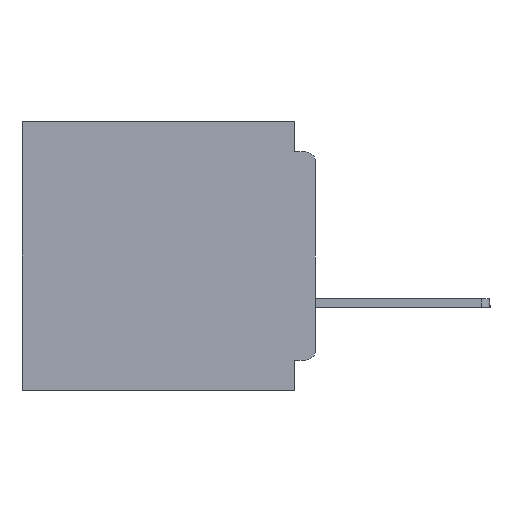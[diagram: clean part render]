
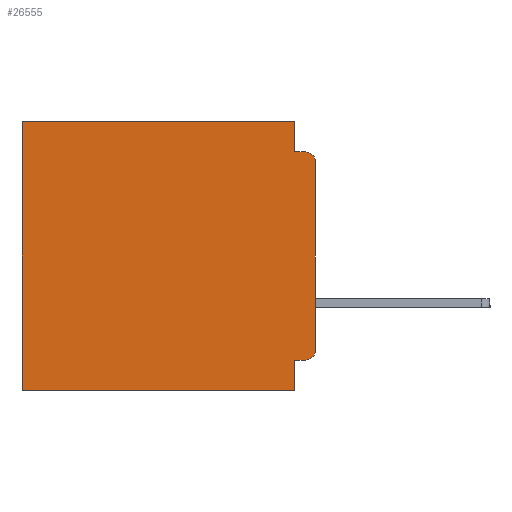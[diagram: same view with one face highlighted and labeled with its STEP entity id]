
A CAD part, left-side view. The second image highlights one B-rep face of the part: STEP entity #26555.
In plain terms, the highlighted planar face has unit normal (-1, 0, 0).
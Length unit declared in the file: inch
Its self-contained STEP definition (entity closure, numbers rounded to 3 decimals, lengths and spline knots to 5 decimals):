
#454 = CARTESIAN_POINT ( 'NONE',  ( 0.3, 0.015, -0.355 ) ) ;
#2407 = ORIENTED_EDGE ( 'NONE', *, *, #19476, .T. ) ;
#2650 = ORIENTED_EDGE ( 'NONE', *, *, #13408, .F. ) ;
#4534 = VECTOR ( 'NONE', #26226, 39.37008 ) ;
#4838 = ORIENTED_EDGE ( 'NONE', *, *, #21185, .T. ) ;
#4865 = VECTOR ( 'NONE', #31657, 39.37008 ) ;
#5301 = EDGE_LOOP ( 'NONE', ( #19419, #4838, #31315, #20966, #7422, #2407, #13477, #11818, #2650, #13776 ) ) ;
#5565 = CARTESIAN_POINT ( 'NONE',  ( 0.3, 0.031, -0.4 ) ) ;
#6075 = EDGE_CURVE ( 'NONE', #13220, #10098, #6987, .T. ) ;
#6446 = AXIS2_PLACEMENT_3D ( 'NONE', #13813, #32935, #16598 ) ;
#6987 = LINE ( 'NONE', #28597, #33619 ) ;
#7422 = ORIENTED_EDGE ( 'NONE', *, *, #6075, .T. ) ;
#8342 = DIRECTION ( 'NONE',  ( 0., 0., -1. ) ) ;
#8594 = VECTOR ( 'NONE', #16568, 39.37008 ) ;
#8645 = CARTESIAN_POINT ( 'NONE',  ( 0.3, 0.437, 0. ) ) ;
#9035 = FACE_OUTER_BOUND ( 'NONE', #5301, .T. ) ;
#9149 = CARTESIAN_POINT ( 'NONE',  ( 0.3, 0., -0.34 ) ) ;
#9679 = EDGE_CURVE ( 'NONE', #10384, #25102, #25056, .T. ) ;
#9707 = CARTESIAN_POINT ( 'NONE',  ( 0.3, 0.031, 0. ) ) ;
#10018 = CARTESIAN_POINT ( 'NONE',  ( 0.3, 0.437, -0.4 ) ) ;
#10098 = VERTEX_POINT ( 'NONE', #8645 ) ;
#10384 = VERTEX_POINT ( 'NONE', #29131 ) ;
#10449 = VECTOR ( 'NONE', #8342, 39.37008 ) ;
#11198 = LINE ( 'NONE', #32913, #8594 ) ;
#11327 = VECTOR ( 'NONE', #35413, 39.37008 ) ;
#11402 = DIRECTION ( 'NONE',  ( -1., 0., 0. ) ) ;
#11818 = ORIENTED_EDGE ( 'NONE', *, *, #19840, .F. ) ;
#11869 = LINE ( 'NONE', #31693, #4534 ) ;
#12404 = CARTESIAN_POINT ( 'NONE',  ( 0.3, 0., -0.4 ) ) ;
#13014 = LINE ( 'NONE', #15460, #20321 ) ;
#13047 = CARTESIAN_POINT ( 'NONE',  ( 0.3, 0., -0.4 ) ) ;
#13220 = VERTEX_POINT ( 'NONE', #34909 ) ;
#13408 = EDGE_CURVE ( 'NONE', #24658, #20834, #11198, .T. ) ;
#13477 = ORIENTED_EDGE ( 'NONE', *, *, #19464, .F. ) ;
#13776 = ORIENTED_EDGE ( 'NONE', *, *, #18913, .T. ) ;
#13813 = CARTESIAN_POINT ( 'NONE',  ( 0.3, 0.015, -0.06 ) ) ;
#13959 = LINE ( 'NONE', #9707, #4865 ) ;
#15460 = CARTESIAN_POINT ( 'NONE',  ( 0.3, 0.031, -0.4 ) ) ;
#15834 = DIRECTION ( 'NONE',  ( 0., 0., -1. ) ) ;
#16134 = VERTEX_POINT ( 'NONE', #29648 ) ;
#16568 = DIRECTION ( 'NONE',  ( 0., 1., 0. ) ) ;
#16598 = DIRECTION ( 'NONE',  ( 0., 0., -1. ) ) ;
#17477 = VERTEX_POINT ( 'NONE', #10018 ) ;
#17479 = AXIS2_PLACEMENT_3D ( 'NONE', #27845, #11402, #30570 ) ;
#18207 = VERTEX_POINT ( 'NONE', #5565 ) ;
#18913 = EDGE_CURVE ( 'NONE', #24658, #25102, #24112, .T. ) ;
#19419 = ORIENTED_EDGE ( 'NONE', *, *, #9679, .F. ) ;
#19464 = EDGE_CURVE ( 'NONE', #18207, #17477, #34023, .T. ) ;
#19476 = EDGE_CURVE ( 'NONE', #10098, #17477, #25930, .T. ) ;
#19840 = EDGE_CURVE ( 'NONE', #20834, #18207, #13014, .T. ) ;
#20321 = VECTOR ( 'NONE', #23673, 39.37008 ) ;
#20834 = VERTEX_POINT ( 'NONE', #31271 ) ;
#20966 = ORIENTED_EDGE ( 'NONE', *, *, #32273, .F. ) ;
#21185 = EDGE_CURVE ( 'NONE', #10384, #26881, #31320, .T. ) ;
#22052 = CARTESIAN_POINT ( 'NONE',  ( 0.3, 0.437, -0.4 ) ) ;
#23673 = DIRECTION ( 'NONE',  ( 0., 0., -1. ) ) ;
#23947 = PLANE ( 'NONE',  #27771 ) ;
#24112 = CIRCLE ( 'NONE', #17479, 0.015 ) ;
#24658 = VERTEX_POINT ( 'NONE', #454 ) ;
#25056 = LINE ( 'NONE', #12404, #33185 ) ;
#25102 = VERTEX_POINT ( 'NONE', #9149 ) ;
#25930 = LINE ( 'NONE', #22052, #10449 ) ;
#26226 = DIRECTION ( 'NONE',  ( 0., -1., 0. ) ) ;
#26555 = ADVANCED_FACE ( 'NONE', ( #9035 ), #23947, .F. ) ;
#26881 = VERTEX_POINT ( 'NONE', #30743 ) ;
#27771 = AXIS2_PLACEMENT_3D ( 'NONE', #13047, #32179, #15834 ) ;
#27845 = CARTESIAN_POINT ( 'NONE',  ( 0.3, 0.015, -0.34 ) ) ;
#28597 = CARTESIAN_POINT ( 'NONE',  ( 0.3, 0., 0. ) ) ;
#29131 = CARTESIAN_POINT ( 'NONE',  ( 0.3, 0., -0.06 ) ) ;
#29648 = CARTESIAN_POINT ( 'NONE',  ( 0.3, 0.031, -0.045 ) ) ;
#29965 = EDGE_CURVE ( 'NONE', #16134, #26881, #11869, .T. ) ;
#30174 = CARTESIAN_POINT ( 'NONE',  ( 0.3, 0., -0.4 ) ) ;
#30570 = DIRECTION ( 'NONE',  ( 0., 0., -1. ) ) ;
#30743 = CARTESIAN_POINT ( 'NONE',  ( 0.3, 0.015, -0.045 ) ) ;
#31271 = CARTESIAN_POINT ( 'NONE',  ( 0.3, 0.031, -0.355 ) ) ;
#31315 = ORIENTED_EDGE ( 'NONE', *, *, #29965, .F. ) ;
#31320 = CIRCLE ( 'NONE', #6446, 0.015 ) ;
#31338 = DIRECTION ( 'NONE',  ( 0., 1., 0. ) ) ;
#31556 = DIRECTION ( 'NONE',  ( 0., 0., -1. ) ) ;
#31657 = DIRECTION ( 'NONE',  ( 0., 0., -1. ) ) ;
#31693 = CARTESIAN_POINT ( 'NONE',  ( 0.3, 0., -0.045 ) ) ;
#32179 = DIRECTION ( 'NONE',  ( 1., 0., 0. ) ) ;
#32273 = EDGE_CURVE ( 'NONE', #13220, #16134, #13959, .T. ) ;
#32913 = CARTESIAN_POINT ( 'NONE',  ( 0.3, 0., -0.355 ) ) ;
#32935 = DIRECTION ( 'NONE',  ( -1., 0., 0. ) ) ;
#33185 = VECTOR ( 'NONE', #31556, 39.37008 ) ;
#33619 = VECTOR ( 'NONE', #31338, 39.37008 ) ;
#34023 = LINE ( 'NONE', #30174, #11327 ) ;
#34909 = CARTESIAN_POINT ( 'NONE',  ( 0.3, 0.031, 0. ) ) ;
#35413 = DIRECTION ( 'NONE',  ( 0., 1., 0. ) ) ;
